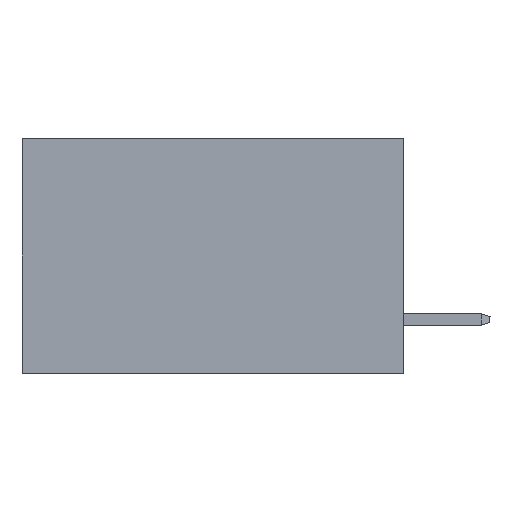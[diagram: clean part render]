
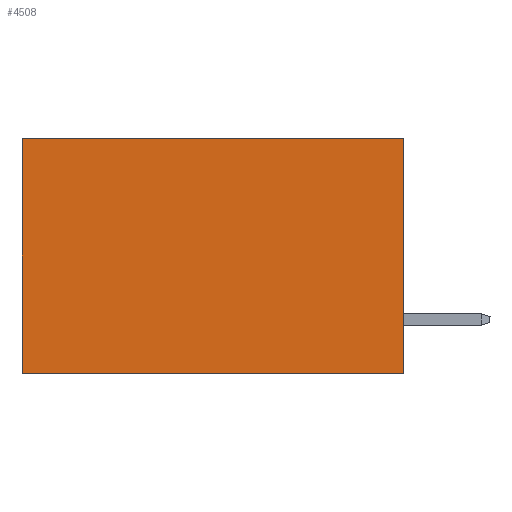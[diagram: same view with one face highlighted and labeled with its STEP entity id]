
A CAD part, left-side view. The second image highlights one B-rep face of the part: STEP entity #4508.
In plain terms, the highlighted planar face has unit normal (-1, 0, 0).
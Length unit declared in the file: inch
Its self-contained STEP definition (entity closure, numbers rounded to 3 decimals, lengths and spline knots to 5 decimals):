
#184 = CARTESIAN_POINT ( 'NONE',  ( 0.2875, 0., 0. ) ) ;
#609 = PLANE ( 'NONE',  #24721 ) ;
#1043 = CARTESIAN_POINT ( 'NONE',  ( 0.2875, 0., 0. ) ) ;
#3153 = DIRECTION ( 'NONE',  ( 0., 1., 0. ) ) ;
#3853 = VECTOR ( 'NONE', #13533, 39.37008 ) ;
#4508 = ADVANCED_FACE ( 'NONE', ( #23465 ), #609, .F. ) ;
#5001 = EDGE_LOOP ( 'NONE', ( #8794, #5338, #11463, #11694 ) ) ;
#5338 = ORIENTED_EDGE ( 'NONE', *, *, #23101, .F. ) ;
#5610 = LINE ( 'NONE', #9677, #3853 ) ;
#6987 = CARTESIAN_POINT ( 'NONE',  ( 0.2875, 0., -0.37 ) ) ;
#7526 = CARTESIAN_POINT ( 'NONE',  ( 0.2875, 0.6, 0. ) ) ;
#8009 = CARTESIAN_POINT ( 'NONE',  ( 0.2875, 0., 0. ) ) ;
#8794 = ORIENTED_EDGE ( 'NONE', *, *, #14921, .T. ) ;
#9677 = CARTESIAN_POINT ( 'NONE',  ( 0.2875, 0., 0. ) ) ;
#11288 = VECTOR ( 'NONE', #3153, 39.37008 ) ;
#11463 = ORIENTED_EDGE ( 'NONE', *, *, #20525, .F. ) ;
#11694 = ORIENTED_EDGE ( 'NONE', *, *, #14335, .T. ) ;
#12903 = DIRECTION ( 'NONE',  ( 0., 0., -1. ) ) ;
#13533 = DIRECTION ( 'NONE',  ( 0., 0., -1. ) ) ;
#14335 = EDGE_CURVE ( 'NONE', #25119, #21176, #21495, .T. ) ;
#14921 = EDGE_CURVE ( 'NONE', #21176, #20055, #23109, .T. ) ;
#15559 = DIRECTION ( 'NONE',  ( 1., 0., 0. ) ) ;
#16239 = CARTESIAN_POINT ( 'NONE',  ( 0.2875, 0.6, 0. ) ) ;
#17205 = LINE ( 'NONE', #6987, #11288 ) ;
#17852 = DIRECTION ( 'NONE',  ( 0., 0., -1. ) ) ;
#19168 = CARTESIAN_POINT ( 'NONE',  ( 0.2875, 0.6, -0.37 ) ) ;
#20055 = VERTEX_POINT ( 'NONE', #19168 ) ;
#20091 = VERTEX_POINT ( 'NONE', #23130 ) ;
#20207 = DIRECTION ( 'NONE',  ( 0., 1., 0. ) ) ;
#20525 = EDGE_CURVE ( 'NONE', #25119, #20091, #5610, .T. ) ;
#21098 = VECTOR ( 'NONE', #12903, 39.37008 ) ;
#21176 = VERTEX_POINT ( 'NONE', #16239 ) ;
#21495 = LINE ( 'NONE', #184, #23116 ) ;
#23101 = EDGE_CURVE ( 'NONE', #20091, #20055, #17205, .T. ) ;
#23109 = LINE ( 'NONE', #7526, #21098 ) ;
#23116 = VECTOR ( 'NONE', #20207, 39.37008 ) ;
#23130 = CARTESIAN_POINT ( 'NONE',  ( 0.2875, 0., -0.37 ) ) ;
#23465 = FACE_OUTER_BOUND ( 'NONE', #5001, .T. ) ;
#24721 = AXIS2_PLACEMENT_3D ( 'NONE', #8009, #15559, #17852 ) ;
#25119 = VERTEX_POINT ( 'NONE', #1043 ) ;
